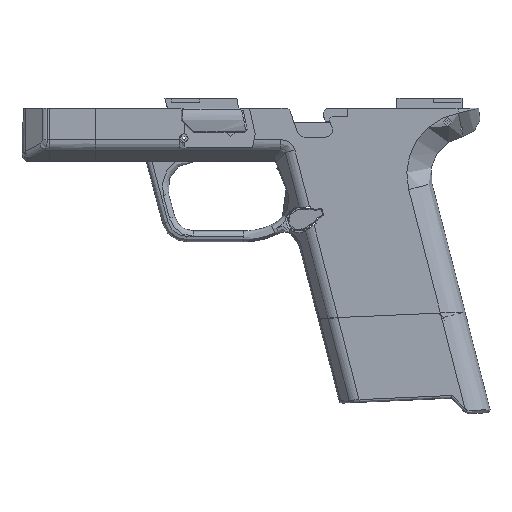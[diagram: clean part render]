
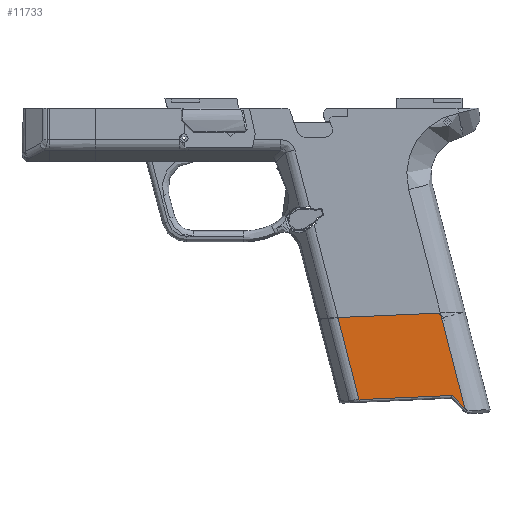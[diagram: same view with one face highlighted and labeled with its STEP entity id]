
A CAD part, left-side view. The second image highlights one B-rep face of the part: STEP entity #11733.
In plain terms, the highlighted face is planar.
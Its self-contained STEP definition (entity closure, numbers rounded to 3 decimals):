
#891=PLANE('',#12886);
#1511=FACE_OUTER_BOUND('',#2179,.T.);
#2179=EDGE_LOOP('',(#10780,#10781,#10782,#10783,#10784));
#3223=LINE('',#22429,#4300);
#3230=LINE('',#22550,#4307);
#3242=LINE('',#22581,#4319);
#3243=LINE('',#22585,#4320);
#3244=LINE('',#22586,#4321);
#4300=VECTOR('',#15916,10.);
#4307=VECTOR('',#15963,10.);
#4319=VECTOR('',#15997,10.);
#4320=VECTOR('',#16002,10.);
#4321=VECTOR('',#16003,10.);
#5715=VERTEX_POINT('',#22261);
#5726=VERTEX_POINT('',#22428);
#5740=VERTEX_POINT('',#22545);
#5748=VERTEX_POINT('',#22580);
#5749=VERTEX_POINT('',#22584);
#7402=EDGE_CURVE('',#5715,#5726,#3223,.T.);
#7425=EDGE_CURVE('',#5726,#5740,#3230,.T.);
#7440=EDGE_CURVE('',#5748,#5740,#3242,.T.);
#7442=EDGE_CURVE('',#5749,#5715,#3243,.T.);
#7443=EDGE_CURVE('',#5749,#5748,#3244,.T.);
#10780=ORIENTED_EDGE('',*,*,#7425,.F.);
#10781=ORIENTED_EDGE('',*,*,#7402,.F.);
#10782=ORIENTED_EDGE('',*,*,#7442,.F.);
#10783=ORIENTED_EDGE('',*,*,#7443,.T.);
#10784=ORIENTED_EDGE('',*,*,#7440,.T.);
#11733=ADVANCED_FACE('',(#1511),#891,.T.);
#12886=AXIS2_PLACEMENT_3D('',#22583,#16000,#16001);
#15916=DIRECTION('',(0.,0.697,-0.717));
#15963=DIRECTION('',(0.,0.999,0.044));
#15997=DIRECTION('',(0.,-0.249,0.969));
#16000=DIRECTION('center_axis',(1.,0.,0.));
#16001=DIRECTION('ref_axis',(0.,0.999,0.044));
#16002=DIRECTION('',(0.,-0.249,0.969));
#16003=DIRECTION('',(0.,0.999,0.044));
#22261=CARTESIAN_POINT('',(22.175,-83.635,101.607));
#22428=CARTESIAN_POINT('',(22.175,-79.055,96.902));
#22429=CARTESIAN_POINT('',(22.175,-73.411,91.103));
#22545=CARTESIAN_POINT('',(22.175,-45.112,98.406));
#22550=CARTESIAN_POINT('',(22.175,-44.983,98.411));
#22580=CARTESIAN_POINT('',(22.175,-37.447,68.587));
#22581=CARTESIAN_POINT('',(22.175,-37.447,68.587));
#22583=CARTESIAN_POINT('Origin',(22.175,-74.722,66.935));
#22584=CARTESIAN_POINT('',(22.175,-74.722,66.935));
#22585=CARTESIAN_POINT('',(22.175,-74.722,66.935));
#22586=CARTESIAN_POINT('',(22.175,-40.785,68.439));
